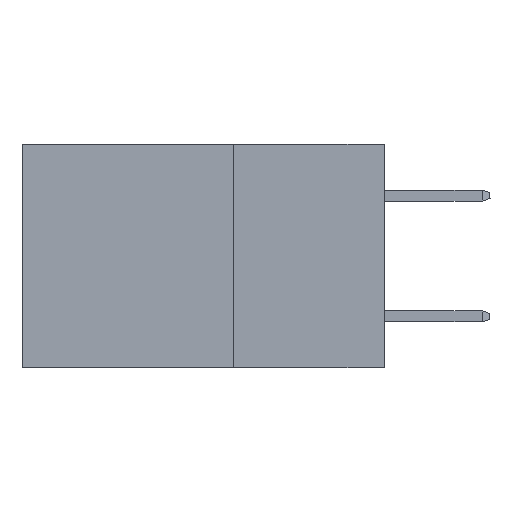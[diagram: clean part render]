
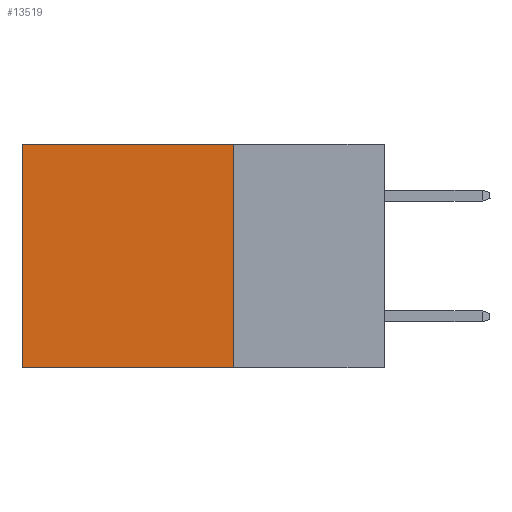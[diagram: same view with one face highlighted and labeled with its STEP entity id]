
A CAD part, left-side view. The second image highlights one B-rep face of the part: STEP entity #13519.
In plain terms, the highlighted planar face has unit normal (-1, 0, 0).
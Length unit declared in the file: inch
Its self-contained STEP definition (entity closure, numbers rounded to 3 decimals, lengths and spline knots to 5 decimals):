
#157 = LINE ( 'NONE', #9767, #17015 ) ;
#653 = EDGE_CURVE ( 'NONE', #20030, #19527, #9757, .T. ) ;
#1275 = DIRECTION ( 'NONE',  ( 1., 0., 0. ) ) ;
#1345 = ORIENTED_EDGE ( 'NONE', *, *, #20627, .F. ) ;
#1616 = DIRECTION ( 'NONE',  ( 0., 1., 0. ) ) ;
#2842 = FACE_OUTER_BOUND ( 'NONE', #4661, .T. ) ;
#3177 = DIRECTION ( 'NONE',  ( 0., 0., -1. ) ) ;
#4155 = VECTOR ( 'NONE', #4480, 39.37008 ) ;
#4451 = ORIENTED_EDGE ( 'NONE', *, *, #12828, .T. ) ;
#4480 = DIRECTION ( 'NONE',  ( 0., 1., 0. ) ) ;
#4661 = EDGE_LOOP ( 'NONE', ( #5886, #1345, #12722, #4451 ) ) ;
#5886 = ORIENTED_EDGE ( 'NONE', *, *, #653, .T. ) ;
#6193 = PLANE ( 'NONE',  #20425 ) ;
#7815 = DIRECTION ( 'NONE',  ( 0., 0., -1. ) ) ;
#8817 = VERTEX_POINT ( 'NONE', #14843 ) ;
#9642 = EDGE_CURVE ( 'NONE', #19271, #8817, #13229, .T. ) ;
#9757 = LINE ( 'NONE', #10147, #14036 ) ;
#9767 = CARTESIAN_POINT ( 'NONE',  ( 0.298, 0.25, -0.37 ) ) ;
#10147 = CARTESIAN_POINT ( 'NONE',  ( 0.298, 0.6, 0. ) ) ;
#10903 = CARTESIAN_POINT ( 'NONE',  ( 0.298, 0.25, 0. ) ) ;
#11264 = CARTESIAN_POINT ( 'NONE',  ( 0.298, 0.25, 0. ) ) ;
#12672 = DIRECTION ( 'NONE',  ( 0., 0., -1. ) ) ;
#12695 = VECTOR ( 'NONE', #3177, 39.37008 ) ;
#12722 = ORIENTED_EDGE ( 'NONE', *, *, #9642, .F. ) ;
#12783 = LINE ( 'NONE', #14189, #4155 ) ;
#12828 = EDGE_CURVE ( 'NONE', #19271, #20030, #12783, .T. ) ;
#13229 = LINE ( 'NONE', #11264, #12695 ) ;
#13519 = ADVANCED_FACE ( 'NONE', ( #2842 ), #6193, .F. ) ;
#14036 = VECTOR ( 'NONE', #7815, 39.37008 ) ;
#14189 = CARTESIAN_POINT ( 'NONE',  ( 0.298, 0.25, 0. ) ) ;
#14843 = CARTESIAN_POINT ( 'NONE',  ( 0.298, 0.25, -0.37 ) ) ;
#16646 = CARTESIAN_POINT ( 'NONE',  ( 0.298, 0.6, -0.37 ) ) ;
#17015 = VECTOR ( 'NONE', #1616, 39.37008 ) ;
#17770 = CARTESIAN_POINT ( 'NONE',  ( 0.298, 0.6, 0. ) ) ;
#19257 = CARTESIAN_POINT ( 'NONE',  ( 0.298, 0.25, 0. ) ) ;
#19271 = VERTEX_POINT ( 'NONE', #19257 ) ;
#19527 = VERTEX_POINT ( 'NONE', #16646 ) ;
#20030 = VERTEX_POINT ( 'NONE', #17770 ) ;
#20425 = AXIS2_PLACEMENT_3D ( 'NONE', #10903, #1275, #12672 ) ;
#20627 = EDGE_CURVE ( 'NONE', #8817, #19527, #157, .T. ) ;
